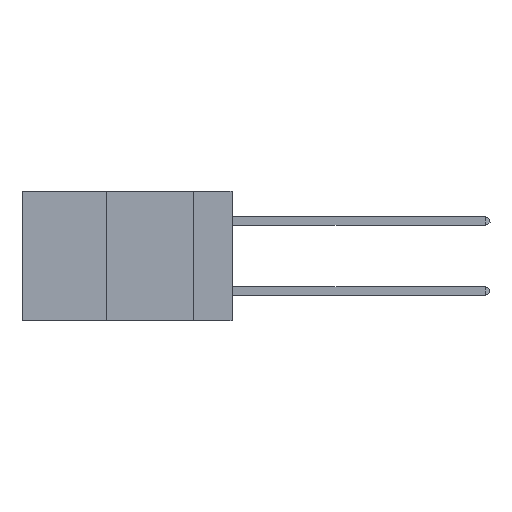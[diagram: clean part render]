
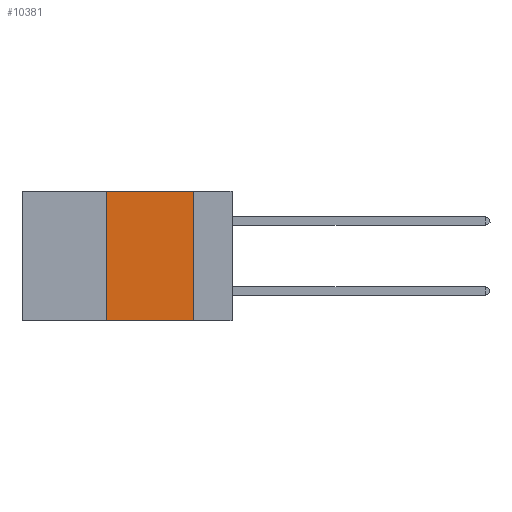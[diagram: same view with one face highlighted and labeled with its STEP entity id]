
A CAD part, left-side view. The second image highlights one B-rep face of the part: STEP entity #10381.
In plain terms, the highlighted planar face has unit normal (-1, 0, 0).
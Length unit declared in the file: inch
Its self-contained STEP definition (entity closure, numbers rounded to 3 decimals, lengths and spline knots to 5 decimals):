
#88 = EDGE_CURVE ( 'NONE', #3147, #16838, #13367, .T. ) ;
#107 = DIRECTION ( 'NONE',  ( 0., 0., -1. ) ) ;
#823 = VERTEX_POINT ( 'NONE', #18046 ) ;
#894 = CARTESIAN_POINT ( 'NONE',  ( 0., 0.6, 0. ) ) ;
#1742 = CARTESIAN_POINT ( 'NONE',  ( 0., 0.36, 0. ) ) ;
#3147 = VERTEX_POINT ( 'NONE', #6670 ) ;
#3630 = EDGE_CURVE ( 'NONE', #16838, #5015, #13216, .T. ) ;
#4112 = ORIENTED_EDGE ( 'NONE', *, *, #88, .F. ) ;
#4118 = CARTESIAN_POINT ( 'NONE',  ( 0., 0.11, 0. ) ) ;
#5015 = VERTEX_POINT ( 'NONE', #4118 ) ;
#5027 = DIRECTION ( 'NONE',  ( 0., 0., 1. ) ) ;
#6098 = DIRECTION ( 'NONE',  ( 1., 0., 0. ) ) ;
#6315 = FACE_OUTER_BOUND ( 'NONE', #21851, .T. ) ;
#6603 = LINE ( 'NONE', #22520, #9030 ) ;
#6670 = CARTESIAN_POINT ( 'NONE',  ( 0., 0.36, -0.37 ) ) ;
#6869 = CARTESIAN_POINT ( 'NONE',  ( 0., 0.36, 0. ) ) ;
#9030 = VECTOR ( 'NONE', #107, 39.37008 ) ;
#9771 = ORIENTED_EDGE ( 'NONE', *, *, #3630, .F. ) ;
#10381 = ADVANCED_FACE ( 'NONE', ( #6315 ), #14790, .F. ) ;
#12325 = DIRECTION ( 'NONE',  ( 0., -1., 0. ) ) ;
#13050 = DIRECTION ( 'NONE',  ( 0., 0., -1. ) ) ;
#13216 = LINE ( 'NONE', #17403, #15387 ) ;
#13367 = LINE ( 'NONE', #6869, #14710 ) ;
#14154 = DIRECTION ( 'NONE',  ( 0., -1., 0. ) ) ;
#14471 = ORIENTED_EDGE ( 'NONE', *, *, #22271, .T. ) ;
#14680 = CARTESIAN_POINT ( 'NONE',  ( 0., 0.6, -0.37 ) ) ;
#14710 = VECTOR ( 'NONE', #5027, 39.37008 ) ;
#14790 = PLANE ( 'NONE',  #20377 ) ;
#15387 = VECTOR ( 'NONE', #12325, 39.37008 ) ;
#16838 = VERTEX_POINT ( 'NONE', #1742 ) ;
#17403 = CARTESIAN_POINT ( 'NONE',  ( 0., 0.6, 0. ) ) ;
#18046 = CARTESIAN_POINT ( 'NONE',  ( 0., 0.11, -0.37 ) ) ;
#19114 = ORIENTED_EDGE ( 'NONE', *, *, #21167, .F. ) ;
#20068 = VECTOR ( 'NONE', #14154, 39.37008 ) ;
#20091 = LINE ( 'NONE', #14680, #20068 ) ;
#20377 = AXIS2_PLACEMENT_3D ( 'NONE', #894, #6098, #13050 ) ;
#21167 = EDGE_CURVE ( 'NONE', #5015, #823, #6603, .T. ) ;
#21851 = EDGE_LOOP ( 'NONE', ( #19114, #9771, #4112, #14471 ) ) ;
#22271 = EDGE_CURVE ( 'NONE', #3147, #823, #20091, .T. ) ;
#22520 = CARTESIAN_POINT ( 'NONE',  ( 0., 0.11, 0. ) ) ;
